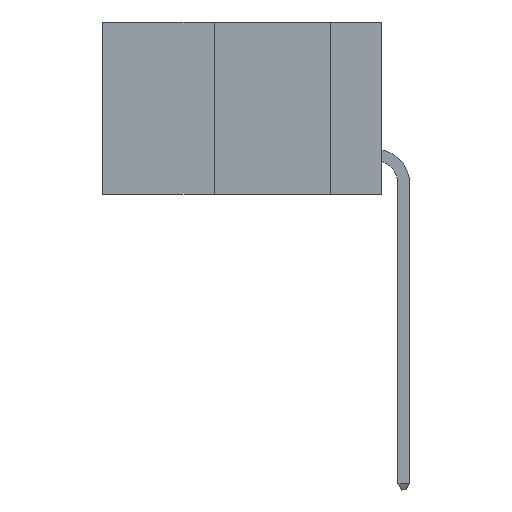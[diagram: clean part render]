
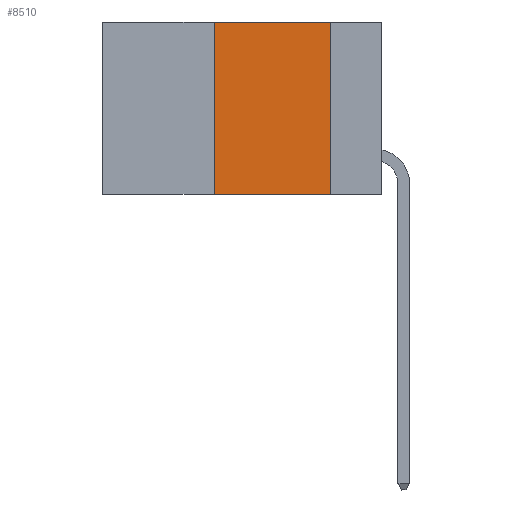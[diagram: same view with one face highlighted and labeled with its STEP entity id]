
A CAD part, left-side view. The second image highlights one B-rep face of the part: STEP entity #8510.
In plain terms, the highlighted planar face has unit normal (-1, 0, 0).
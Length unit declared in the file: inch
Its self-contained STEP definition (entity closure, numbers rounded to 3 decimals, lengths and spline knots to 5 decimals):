
#435 = ORIENTED_EDGE ( 'NONE', *, *, #1361, .F. ) ;
#1045 = DIRECTION ( 'NONE',  ( 0., -1., 0. ) ) ;
#1267 = CARTESIAN_POINT ( 'NONE',  ( 0., 0.11, 0. ) ) ;
#1361 = EDGE_CURVE ( 'NONE', #1857, #9229, #5022, .T. ) ;
#1793 = CARTESIAN_POINT ( 'NONE',  ( 0., 0.6, 0. ) ) ;
#1857 = VERTEX_POINT ( 'NONE', #7605 ) ;
#2067 = CARTESIAN_POINT ( 'NONE',  ( 0., 0.11, 0. ) ) ;
#2692 = CARTESIAN_POINT ( 'NONE',  ( 0., 0.6, -0.37 ) ) ;
#2987 = CARTESIAN_POINT ( 'NONE',  ( 0., 0.6, 0. ) ) ;
#3000 = EDGE_LOOP ( 'NONE', ( #9988, #435, #11143, #4871 ) ) ;
#3310 = VERTEX_POINT ( 'NONE', #9420 ) ;
#4288 = EDGE_CURVE ( 'NONE', #9229, #3310, #4320, .T. ) ;
#4320 = LINE ( 'NONE', #2067, #9662 ) ;
#4405 = LINE ( 'NONE', #2692, #9741 ) ;
#4509 = CARTESIAN_POINT ( 'NONE',  ( 0., 0.36, -0.37 ) ) ;
#4675 = EDGE_CURVE ( 'NONE', #9459, #1857, #8383, .T. ) ;
#4871 = ORIENTED_EDGE ( 'NONE', *, *, #9864, .T. ) ;
#4906 = DIRECTION ( 'NONE',  ( 0., 0., 1. ) ) ;
#5022 = LINE ( 'NONE', #2987, #10225 ) ;
#6430 = DIRECTION ( 'NONE',  ( 0., -1., 0. ) ) ;
#6465 = DIRECTION ( 'NONE',  ( 0., 0., -1. ) ) ;
#6750 = CARTESIAN_POINT ( 'NONE',  ( 0., 0.36, 0. ) ) ;
#6834 = FACE_OUTER_BOUND ( 'NONE', #3000, .T. ) ;
#7110 = AXIS2_PLACEMENT_3D ( 'NONE', #1793, #12019, #6465 ) ;
#7605 = CARTESIAN_POINT ( 'NONE',  ( 0., 0.36, 0. ) ) ;
#7651 = VECTOR ( 'NONE', #4906, 39.37008 ) ;
#8383 = LINE ( 'NONE', #6750, #7651 ) ;
#8510 = ADVANCED_FACE ( 'NONE', ( #6834 ), #8768, .F. ) ;
#8768 = PLANE ( 'NONE',  #7110 ) ;
#9229 = VERTEX_POINT ( 'NONE', #1267 ) ;
#9420 = CARTESIAN_POINT ( 'NONE',  ( 0., 0.11, -0.37 ) ) ;
#9459 = VERTEX_POINT ( 'NONE', #4509 ) ;
#9662 = VECTOR ( 'NONE', #10339, 39.37008 ) ;
#9741 = VECTOR ( 'NONE', #6430, 39.37008 ) ;
#9864 = EDGE_CURVE ( 'NONE', #9459, #3310, #4405, .T. ) ;
#9988 = ORIENTED_EDGE ( 'NONE', *, *, #4288, .F. ) ;
#10225 = VECTOR ( 'NONE', #1045, 39.37008 ) ;
#10339 = DIRECTION ( 'NONE',  ( 0., 0., -1. ) ) ;
#11143 = ORIENTED_EDGE ( 'NONE', *, *, #4675, .F. ) ;
#12019 = DIRECTION ( 'NONE',  ( 1., 0., 0. ) ) ;
